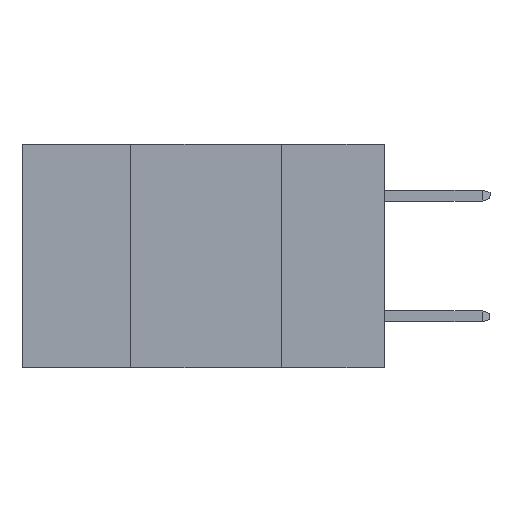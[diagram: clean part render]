
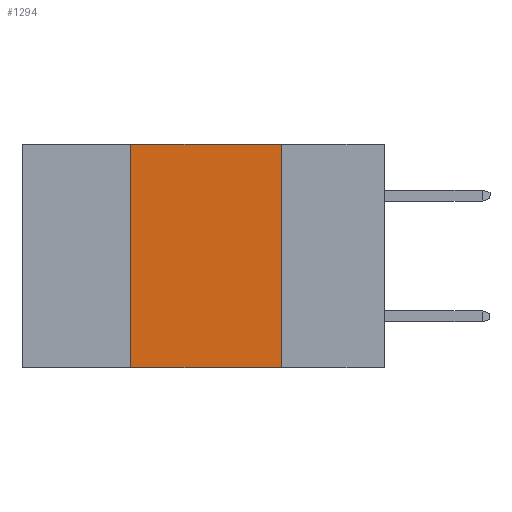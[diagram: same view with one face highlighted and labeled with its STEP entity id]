
A CAD part, left-side view. The second image highlights one B-rep face of the part: STEP entity #1294.
In plain terms, the highlighted planar face has unit normal (-1, 0, 0).
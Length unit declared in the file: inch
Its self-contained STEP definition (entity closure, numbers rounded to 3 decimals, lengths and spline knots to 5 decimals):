
#45 = EDGE_CURVE ( 'NONE', #8423, #6369, #5813, .T. ) ;
#428 = CARTESIAN_POINT ( 'NONE',  ( 0., 0.6, -0.37 ) ) ;
#549 = EDGE_CURVE ( 'NONE', #6822, #6369, #2459, .T. ) ;
#577 = EDGE_CURVE ( 'NONE', #5315, #6822, #3013, .T. ) ;
#588 = DIRECTION ( 'NONE',  ( 0., -1., 0. ) ) ;
#956 = DIRECTION ( 'NONE',  ( 0., 0., -1. ) ) ;
#1216 = CARTESIAN_POINT ( 'NONE',  ( 0., 0.6, 0. ) ) ;
#1294 = ADVANCED_FACE ( 'NONE', ( #3682 ), #6417, .F. ) ;
#1667 = ORIENTED_EDGE ( 'NONE', *, *, #3636, .F. ) ;
#1695 = DIRECTION ( 'NONE',  ( 0., 0., -1. ) ) ;
#1743 = CARTESIAN_POINT ( 'NONE',  ( 0., 0.6, 0. ) ) ;
#2013 = VECTOR ( 'NONE', #8573, 39.37008 ) ;
#2114 = LINE ( 'NONE', #5310, #5220 ) ;
#2375 = CARTESIAN_POINT ( 'NONE',  ( 0., 0.17, -0.37 ) ) ;
#2459 = LINE ( 'NONE', #2375, #7742 ) ;
#3013 = LINE ( 'NONE', #1216, #5929 ) ;
#3636 = EDGE_CURVE ( 'NONE', #8423, #5315, #2114, .T. ) ;
#3682 = FACE_OUTER_BOUND ( 'NONE', #5657, .T. ) ;
#3771 = CARTESIAN_POINT ( 'NONE',  ( 0., 0.17, 0. ) ) ;
#4336 = ORIENTED_EDGE ( 'NONE', *, *, #577, .F. ) ;
#4420 = AXIS2_PLACEMENT_3D ( 'NONE', #1743, #7181, #956 ) ;
#5220 = VECTOR ( 'NONE', #8007, 39.37008 ) ;
#5256 = CARTESIAN_POINT ( 'NONE',  ( 0., 0.42, -0.37 ) ) ;
#5310 = CARTESIAN_POINT ( 'NONE',  ( 0., 0.42, -0.37 ) ) ;
#5315 = VERTEX_POINT ( 'NONE', #7354 ) ;
#5603 = ORIENTED_EDGE ( 'NONE', *, *, #45, .T. ) ;
#5635 = CARTESIAN_POINT ( 'NONE',  ( 0., 0.17, -0.37 ) ) ;
#5657 = EDGE_LOOP ( 'NONE', ( #8011, #4336, #1667, #5603 ) ) ;
#5813 = LINE ( 'NONE', #428, #2013 ) ;
#5929 = VECTOR ( 'NONE', #588, 39.37008 ) ;
#6369 = VERTEX_POINT ( 'NONE', #5635 ) ;
#6417 = PLANE ( 'NONE',  #4420 ) ;
#6822 = VERTEX_POINT ( 'NONE', #3771 ) ;
#7181 = DIRECTION ( 'NONE',  ( 1., 0., 0. ) ) ;
#7354 = CARTESIAN_POINT ( 'NONE',  ( 0., 0.42, 0. ) ) ;
#7742 = VECTOR ( 'NONE', #1695, 39.37008 ) ;
#8007 = DIRECTION ( 'NONE',  ( 0., 0., 1. ) ) ;
#8011 = ORIENTED_EDGE ( 'NONE', *, *, #549, .F. ) ;
#8423 = VERTEX_POINT ( 'NONE', #5256 ) ;
#8573 = DIRECTION ( 'NONE',  ( 0., -1., 0. ) ) ;
